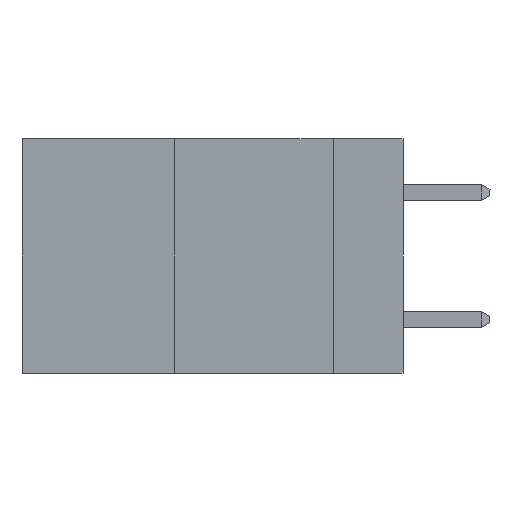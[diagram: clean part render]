
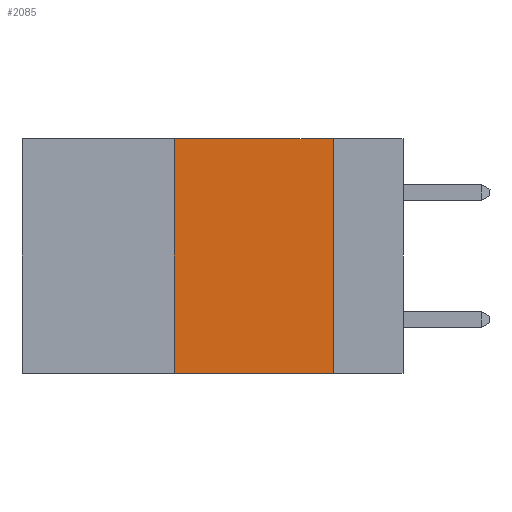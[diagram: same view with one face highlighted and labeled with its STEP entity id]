
A CAD part, left-side view. The second image highlights one B-rep face of the part: STEP entity #2085.
In plain terms, the highlighted planar face has unit normal (-1, 0, 0).
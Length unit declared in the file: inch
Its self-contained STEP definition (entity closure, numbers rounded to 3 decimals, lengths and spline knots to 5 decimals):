
#214 = EDGE_CURVE ( 'NONE', #9570, #12347, #3585, .T. ) ;
#677 = ORIENTED_EDGE ( 'NONE', *, *, #6858, .F. ) ;
#1292 = EDGE_LOOP ( 'NONE', ( #677, #1529, #5542, #3835 ) ) ;
#1488 = DIRECTION ( 'NONE',  ( 1., 0., 0. ) ) ;
#1529 = ORIENTED_EDGE ( 'NONE', *, *, #214, .F. ) ;
#2085 = ADVANCED_FACE ( 'NONE', ( #3326 ), #12585, .F. ) ;
#2815 = CARTESIAN_POINT ( 'NONE',  ( 0., 0.6, 0. ) ) ;
#3326 = FACE_OUTER_BOUND ( 'NONE', #1292, .T. ) ;
#3585 = LINE ( 'NONE', #4050, #9133 ) ;
#3835 = ORIENTED_EDGE ( 'NONE', *, *, #4582, .T. ) ;
#4050 = CARTESIAN_POINT ( 'NONE',  ( 0., 0.6, 0. ) ) ;
#4119 = VECTOR ( 'NONE', #12038, 39.37008 ) ;
#4434 = CARTESIAN_POINT ( 'NONE',  ( 0., 0.36, -0.37 ) ) ;
#4582 = EDGE_CURVE ( 'NONE', #12990, #7994, #9985, .T. ) ;
#4620 = VECTOR ( 'NONE', #14090, 39.37008 ) ;
#4760 = VECTOR ( 'NONE', #5617, 39.37008 ) ;
#5368 = EDGE_CURVE ( 'NONE', #12990, #9570, #7263, .T. ) ;
#5380 = CARTESIAN_POINT ( 'NONE',  ( 0., 0.11, -0.37 ) ) ;
#5542 = ORIENTED_EDGE ( 'NONE', *, *, #5368, .F. ) ;
#5617 = DIRECTION ( 'NONE',  ( 0., 0., -1. ) ) ;
#5633 = CARTESIAN_POINT ( 'NONE',  ( 0., 0.6, -0.37 ) ) ;
#6065 = DIRECTION ( 'NONE',  ( 0., -1., 0. ) ) ;
#6858 = EDGE_CURVE ( 'NONE', #12347, #7994, #10577, .T. ) ;
#7263 = LINE ( 'NONE', #7814, #4620 ) ;
#7766 = CARTESIAN_POINT ( 'NONE',  ( 0., 0.11, 0. ) ) ;
#7814 = CARTESIAN_POINT ( 'NONE',  ( 0., 0.36, 0. ) ) ;
#7960 = DIRECTION ( 'NONE',  ( 0., 0., -1. ) ) ;
#7994 = VERTEX_POINT ( 'NONE', #5380 ) ;
#9133 = VECTOR ( 'NONE', #6065, 39.37008 ) ;
#9570 = VERTEX_POINT ( 'NONE', #13687 ) ;
#9985 = LINE ( 'NONE', #5633, #4119 ) ;
#10106 = AXIS2_PLACEMENT_3D ( 'NONE', #2815, #1488, #7960 ) ;
#10577 = LINE ( 'NONE', #7766, #4760 ) ;
#12038 = DIRECTION ( 'NONE',  ( 0., -1., 0. ) ) ;
#12347 = VERTEX_POINT ( 'NONE', #13454 ) ;
#12585 = PLANE ( 'NONE',  #10106 ) ;
#12990 = VERTEX_POINT ( 'NONE', #4434 ) ;
#13454 = CARTESIAN_POINT ( 'NONE',  ( 0., 0.11, 0. ) ) ;
#13687 = CARTESIAN_POINT ( 'NONE',  ( 0., 0.36, 0. ) ) ;
#14090 = DIRECTION ( 'NONE',  ( 0., 0., 1. ) ) ;
